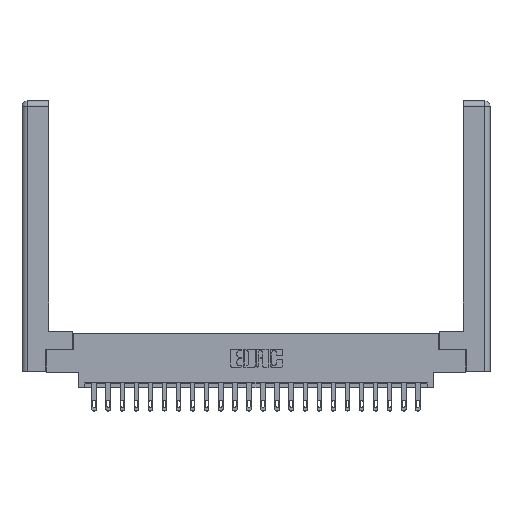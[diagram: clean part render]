
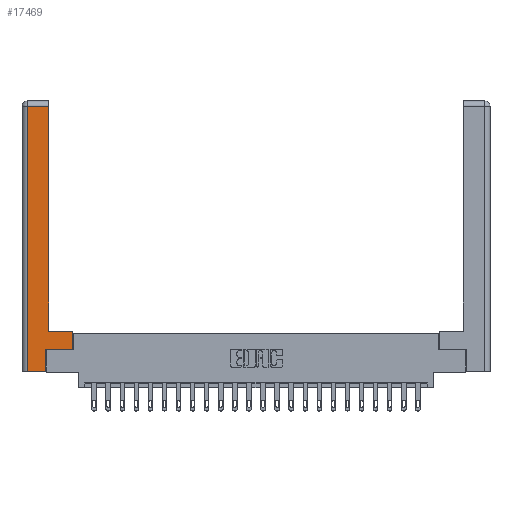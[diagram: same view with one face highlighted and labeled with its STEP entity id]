
A CAD part, top view. The second image highlights one B-rep face of the part: STEP entity #17469.
In plain terms, the highlighted planar face has unit normal (0, 0, 1).
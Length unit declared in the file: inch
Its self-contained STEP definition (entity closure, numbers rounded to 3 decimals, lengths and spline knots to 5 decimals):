
#105 = VERTEX_POINT ( 'NONE', #17931 ) ;
#214 = DIRECTION ( 'NONE',  ( -1., 0., 0. ) ) ;
#703 = CARTESIAN_POINT ( 'NONE',  ( 0.565, 0.45, 0. ) ) ;
#863 = LINE ( 'NONE', #12072, #2276 ) ;
#938 = CARTESIAN_POINT ( 'NONE',  ( 0.565, 0.245, 0. ) ) ;
#1812 = CARTESIAN_POINT ( 'NONE',  ( 0., 0., 0. ) ) ;
#1935 = CARTESIAN_POINT ( 'NONE',  ( 0.565, 0.245, 0. ) ) ;
#2177 = VECTOR ( 'NONE', #8282, 39.37008 ) ;
#2276 = VECTOR ( 'NONE', #13913, 39.37008 ) ;
#2738 = EDGE_CURVE ( 'NONE', #19079, #3175, #12440, .T. ) ;
#2762 = ORIENTED_EDGE ( 'NONE', *, *, #21759, .T. ) ;
#3175 = VERTEX_POINT ( 'NONE', #5705 ) ;
#3300 = LINE ( 'NONE', #17411, #2177 ) ;
#3609 = EDGE_CURVE ( 'NONE', #4370, #16451, #14683, .T. ) ;
#3709 = VECTOR ( 'NONE', #18998, 39.37008 ) ;
#4370 = VERTEX_POINT ( 'NONE', #9066 ) ;
#4470 = LINE ( 'NONE', #13828, #15952 ) ;
#4749 = ORIENTED_EDGE ( 'NONE', *, *, #2738, .T. ) ;
#5580 = CARTESIAN_POINT ( 'NONE',  ( 0.295, 0.45, 0. ) ) ;
#5705 = CARTESIAN_POINT ( 'NONE',  ( 0.0615, 2.94, 0. ) ) ;
#6433 = CARTESIAN_POINT ( 'NONE',  ( 0.0615, 2.94, 0. ) ) ;
#6849 = LINE ( 'NONE', #13446, #3709 ) ;
#7310 = CARTESIAN_POINT ( 'NONE',  ( 0.265, 0.245, 0. ) ) ;
#7714 = EDGE_CURVE ( 'NONE', #22550, #19079, #3300, .T. ) ;
#8152 = DIRECTION ( 'NONE',  ( 0., 1., 0. ) ) ;
#8282 = DIRECTION ( 'NONE',  ( 0., 1., 0. ) ) ;
#8797 = VECTOR ( 'NONE', #13492, 39.37008 ) ;
#9066 = CARTESIAN_POINT ( 'NONE',  ( 0.265, 0.245, 0. ) ) ;
#9287 = FACE_OUTER_BOUND ( 'NONE', #22455, .T. ) ;
#10969 = VECTOR ( 'NONE', #21906, 39.37008 ) ;
#12072 = CARTESIAN_POINT ( 'NONE',  ( 0.0615, 0., 0. ) ) ;
#12152 = EDGE_CURVE ( 'NONE', #105, #16611, #6849, .T. ) ;
#12262 = EDGE_CURVE ( 'NONE', #3175, #105, #863, .T. ) ;
#12398 = ORIENTED_EDGE ( 'NONE', *, *, #22510, .T. ) ;
#12440 = LINE ( 'NONE', #6433, #22724 ) ;
#12465 = LINE ( 'NONE', #7310, #13038 ) ;
#12750 = PLANE ( 'NONE',  #13825 ) ;
#13038 = VECTOR ( 'NONE', #13989, 39.37008 ) ;
#13446 = CARTESIAN_POINT ( 'NONE',  ( 0.265, 0., 0. ) ) ;
#13492 = DIRECTION ( 'NONE',  ( -1., 0., 0. ) ) ;
#13741 = DIRECTION ( 'NONE',  ( -1., 0., 0. ) ) ;
#13804 = CARTESIAN_POINT ( 'NONE',  ( 0.295, 0.45, 0. ) ) ;
#13825 = AXIS2_PLACEMENT_3D ( 'NONE', #1812, #14584, #214 ) ;
#13828 = CARTESIAN_POINT ( 'NONE',  ( 0.565, 0.45, 0. ) ) ;
#13913 = DIRECTION ( 'NONE',  ( 0., -1., 0. ) ) ;
#13989 = DIRECTION ( 'NONE',  ( 0., 1., 0. ) ) ;
#13995 = ORIENTED_EDGE ( 'NONE', *, *, #3609, .T. ) ;
#14114 = ORIENTED_EDGE ( 'NONE', *, *, #12152, .T. ) ;
#14584 = DIRECTION ( 'NONE',  ( 0., 0., -1. ) ) ;
#14683 = LINE ( 'NONE', #1935, #10969 ) ;
#15318 = EDGE_CURVE ( 'NONE', #18160, #22550, #21103, .T. ) ;
#15952 = VECTOR ( 'NONE', #8152, 39.37008 ) ;
#16451 = VERTEX_POINT ( 'NONE', #938 ) ;
#16611 = VERTEX_POINT ( 'NONE', #23599 ) ;
#17411 = CARTESIAN_POINT ( 'NONE',  ( 0.295, 3., 0. ) ) ;
#17469 = ADVANCED_FACE ( 'NONE', ( #9287 ), #12750, .F. ) ;
#17931 = CARTESIAN_POINT ( 'NONE',  ( 0.0615, 0., 0. ) ) ;
#18032 = CARTESIAN_POINT ( 'NONE',  ( 0.295, 2.94, 0. ) ) ;
#18160 = VERTEX_POINT ( 'NONE', #703 ) ;
#18998 = DIRECTION ( 'NONE',  ( 1., 0., 0. ) ) ;
#19079 = VERTEX_POINT ( 'NONE', #18032 ) ;
#19430 = ORIENTED_EDGE ( 'NONE', *, *, #7714, .T. ) ;
#20965 = ORIENTED_EDGE ( 'NONE', *, *, #15318, .T. ) ;
#21103 = LINE ( 'NONE', #13804, #8797 ) ;
#21759 = EDGE_CURVE ( 'NONE', #16451, #18160, #4470, .T. ) ;
#21906 = DIRECTION ( 'NONE',  ( 1., 0., 0. ) ) ;
#22455 = EDGE_LOOP ( 'NONE', ( #19430, #4749, #22644, #14114, #12398, #13995, #2762, #20965 ) ) ;
#22510 = EDGE_CURVE ( 'NONE', #16611, #4370, #12465, .T. ) ;
#22550 = VERTEX_POINT ( 'NONE', #5580 ) ;
#22644 = ORIENTED_EDGE ( 'NONE', *, *, #12262, .T. ) ;
#22724 = VECTOR ( 'NONE', #13741, 39.37008 ) ;
#23599 = CARTESIAN_POINT ( 'NONE',  ( 0.265, 0., 0. ) ) ;
